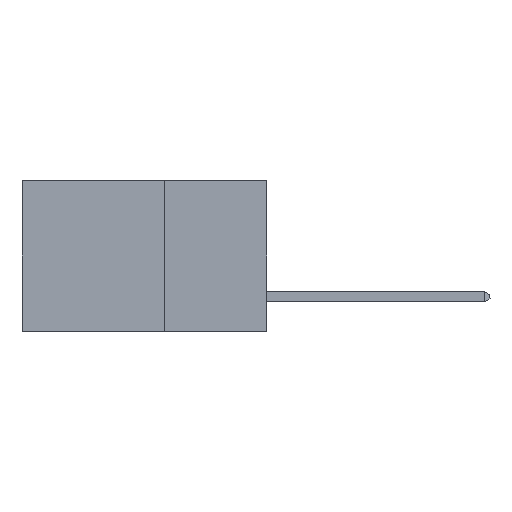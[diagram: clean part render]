
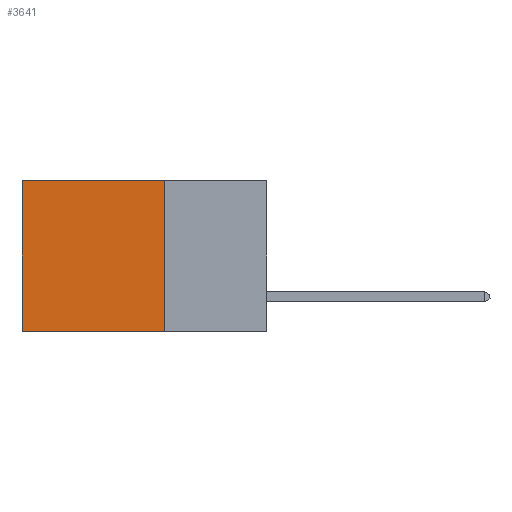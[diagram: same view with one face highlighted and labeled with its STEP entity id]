
A CAD part, left-side view. The second image highlights one B-rep face of the part: STEP entity #3641.
In plain terms, the highlighted planar face has unit normal (-1, 0, 0).
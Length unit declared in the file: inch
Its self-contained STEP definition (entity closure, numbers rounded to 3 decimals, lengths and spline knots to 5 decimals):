
#81 = VECTOR ( 'NONE', #10286, 39.37008 ) ;
#100 = EDGE_LOOP ( 'NONE', ( #9963, #8094, #3030, #8658 ) ) ;
#318 = DIRECTION ( 'NONE',  ( 0., 1., 0. ) ) ;
#763 = VERTEX_POINT ( 'NONE', #9283 ) ;
#786 = PLANE ( 'NONE',  #2343 ) ;
#865 = LINE ( 'NONE', #9898, #4977 ) ;
#1103 = VERTEX_POINT ( 'NONE', #7716 ) ;
#1453 = CARTESIAN_POINT ( 'NONE',  ( 0.2875, 0.6, 0. ) ) ;
#2343 = AXIS2_PLACEMENT_3D ( 'NONE', #15819, #9659, #12114 ) ;
#2617 = DIRECTION ( 'NONE',  ( 0., 1., 0. ) ) ;
#3030 = ORIENTED_EDGE ( 'NONE', *, *, #11470, .F. ) ;
#3641 = ADVANCED_FACE ( 'NONE', ( #10105 ), #786, .F. ) ;
#3923 = LINE ( 'NONE', #8436, #11138 ) ;
#4499 = CARTESIAN_POINT ( 'NONE',  ( 0.2875, 0.25, 0. ) ) ;
#4977 = VECTOR ( 'NONE', #2617, 39.37008 ) ;
#6544 = LINE ( 'NONE', #1453, #81 ) ;
#7167 = VERTEX_POINT ( 'NONE', #12938 ) ;
#7716 = CARTESIAN_POINT ( 'NONE',  ( 0.2875, 0.25, 0. ) ) ;
#8094 = ORIENTED_EDGE ( 'NONE', *, *, #16172, .F. ) ;
#8238 = DIRECTION ( 'NONE',  ( 0., 0., -1. ) ) ;
#8276 = VERTEX_POINT ( 'NONE', #14409 ) ;
#8436 = CARTESIAN_POINT ( 'NONE',  ( 0.2875, 0.25, -0.37 ) ) ;
#8658 = ORIENTED_EDGE ( 'NONE', *, *, #8971, .T. ) ;
#8971 = EDGE_CURVE ( 'NONE', #1103, #763, #865, .T. ) ;
#9283 = CARTESIAN_POINT ( 'NONE',  ( 0.2875, 0.6, 0. ) ) ;
#9431 = LINE ( 'NONE', #4499, #13865 ) ;
#9659 = DIRECTION ( 'NONE',  ( 1., 0., 0. ) ) ;
#9898 = CARTESIAN_POINT ( 'NONE',  ( 0.2875, 0.25, 0. ) ) ;
#9963 = ORIENTED_EDGE ( 'NONE', *, *, #13983, .T. ) ;
#10105 = FACE_OUTER_BOUND ( 'NONE', #100, .T. ) ;
#10286 = DIRECTION ( 'NONE',  ( 0., 0., -1. ) ) ;
#11138 = VECTOR ( 'NONE', #318, 39.37008 ) ;
#11470 = EDGE_CURVE ( 'NONE', #1103, #7167, #9431, .T. ) ;
#12114 = DIRECTION ( 'NONE',  ( 0., 0., -1. ) ) ;
#12938 = CARTESIAN_POINT ( 'NONE',  ( 0.2875, 0.25, -0.37 ) ) ;
#13865 = VECTOR ( 'NONE', #8238, 39.37008 ) ;
#13983 = EDGE_CURVE ( 'NONE', #763, #8276, #6544, .T. ) ;
#14409 = CARTESIAN_POINT ( 'NONE',  ( 0.2875, 0.6, -0.37 ) ) ;
#15819 = CARTESIAN_POINT ( 'NONE',  ( 0.2875, 0.25, 0. ) ) ;
#16172 = EDGE_CURVE ( 'NONE', #7167, #8276, #3923, .T. ) ;
